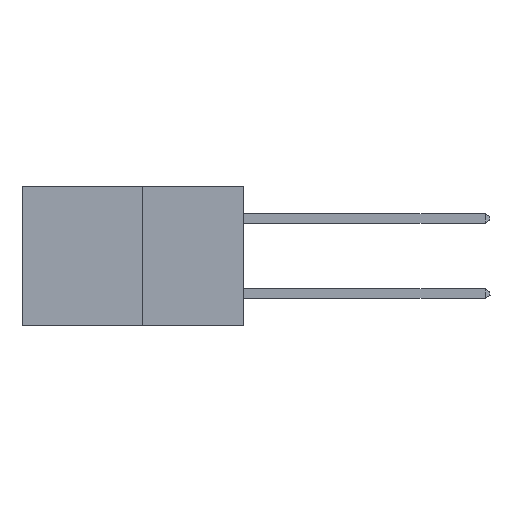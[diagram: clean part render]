
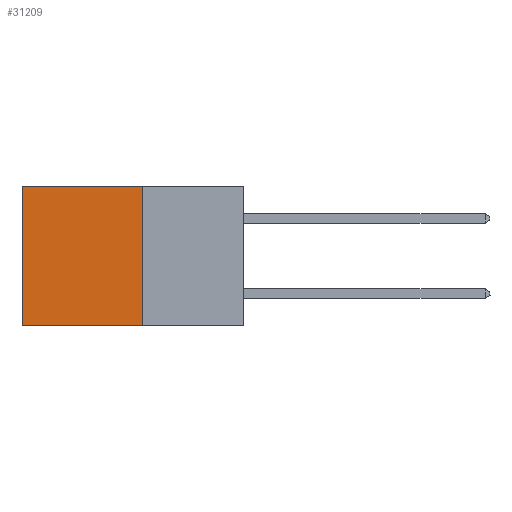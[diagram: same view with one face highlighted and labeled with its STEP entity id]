
A CAD part, left-side view. The second image highlights one B-rep face of the part: STEP entity #31209.
In plain terms, the highlighted planar face has unit normal (-1, 0, 0).
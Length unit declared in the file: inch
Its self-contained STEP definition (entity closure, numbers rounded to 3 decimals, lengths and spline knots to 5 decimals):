
#538 = LINE ( 'NONE', #18435, #14030 ) ;
#1181 = LINE ( 'NONE', #32387, #28103 ) ;
#3532 = EDGE_CURVE ( 'NONE', #28994, #14447, #1181, .T. ) ;
#6191 = CARTESIAN_POINT ( 'NONE',  ( 0.277, 0.59, 0. ) ) ;
#8257 = VERTEX_POINT ( 'NONE', #15634 ) ;
#8579 = VERTEX_POINT ( 'NONE', #6191 ) ;
#10145 = PLANE ( 'NONE',  #22288 ) ;
#11456 = EDGE_CURVE ( 'NONE', #28994, #8579, #32967, .T. ) ;
#14030 = VECTOR ( 'NONE', #29262, 39.37008 ) ;
#14278 = VECTOR ( 'NONE', #18997, 39.37008 ) ;
#14447 = VERTEX_POINT ( 'NONE', #17115 ) ;
#15563 = DIRECTION ( 'NONE',  ( 0., 0., -1. ) ) ;
#15634 = CARTESIAN_POINT ( 'NONE',  ( 0.277, 0.59, -0.37 ) ) ;
#16343 = CARTESIAN_POINT ( 'NONE',  ( 0.277, 0.27, -0.37 ) ) ;
#17115 = CARTESIAN_POINT ( 'NONE',  ( 0.277, 0.27, -0.37 ) ) ;
#18435 = CARTESIAN_POINT ( 'NONE',  ( 0.277, 0.59, -0.37 ) ) ;
#18654 = VECTOR ( 'NONE', #24151, 39.37008 ) ;
#18997 = DIRECTION ( 'NONE',  ( 0., 1., 0. ) ) ;
#19193 = EDGE_CURVE ( 'NONE', #14447, #8257, #27692, .T. ) ;
#21454 = CARTESIAN_POINT ( 'NONE',  ( 0.277, 0.27, 0. ) ) ;
#22288 = AXIS2_PLACEMENT_3D ( 'NONE', #28936, #31648, #15563 ) ;
#22805 = ORIENTED_EDGE ( 'NONE', *, *, #3532, .F. ) ;
#23451 = EDGE_LOOP ( 'NONE', ( #23962, #26553, #22805, #31259 ) ) ;
#23962 = ORIENTED_EDGE ( 'NONE', *, *, #29102, .T. ) ;
#24151 = DIRECTION ( 'NONE',  ( 0., 1., 0. ) ) ;
#26553 = ORIENTED_EDGE ( 'NONE', *, *, #19193, .F. ) ;
#27692 = LINE ( 'NONE', #16343, #14278 ) ;
#28103 = VECTOR ( 'NONE', #32195, 39.37008 ) ;
#28797 = CARTESIAN_POINT ( 'NONE',  ( 0.277, 0.27, 0. ) ) ;
#28936 = CARTESIAN_POINT ( 'NONE',  ( 0.277, 0.27, -0.37 ) ) ;
#28994 = VERTEX_POINT ( 'NONE', #28797 ) ;
#29102 = EDGE_CURVE ( 'NONE', #8579, #8257, #538, .T. ) ;
#29262 = DIRECTION ( 'NONE',  ( 0., 0., -1. ) ) ;
#31209 = ADVANCED_FACE ( 'NONE', ( #32303 ), #10145, .F. ) ;
#31259 = ORIENTED_EDGE ( 'NONE', *, *, #11456, .T. ) ;
#31648 = DIRECTION ( 'NONE',  ( 1., 0., 0. ) ) ;
#32195 = DIRECTION ( 'NONE',  ( 0., 0., -1. ) ) ;
#32303 = FACE_OUTER_BOUND ( 'NONE', #23451, .T. ) ;
#32387 = CARTESIAN_POINT ( 'NONE',  ( 0.277, 0.27, -0.37 ) ) ;
#32967 = LINE ( 'NONE', #21454, #18654 ) ;
